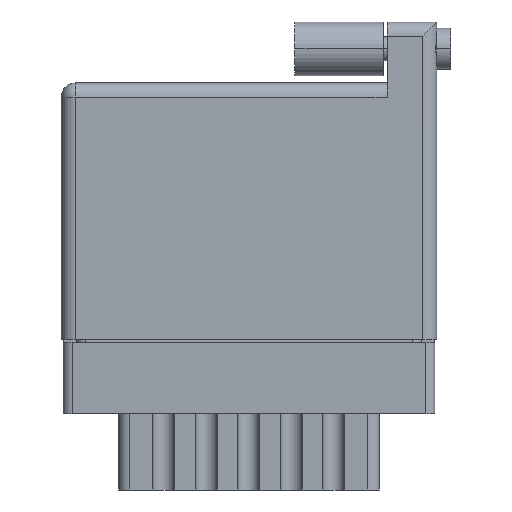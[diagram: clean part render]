
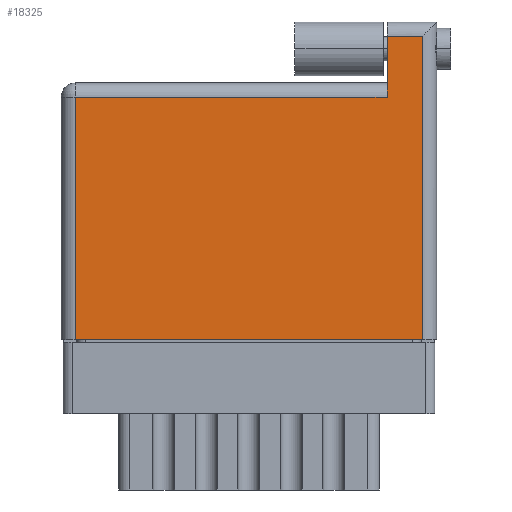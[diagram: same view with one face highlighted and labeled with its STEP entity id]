
A CAD part, front view. The second image highlights one B-rep face of the part: STEP entity #18325.
In plain terms, the highlighted face is planar.
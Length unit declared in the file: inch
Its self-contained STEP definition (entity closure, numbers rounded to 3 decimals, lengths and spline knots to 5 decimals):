
#205 = VECTOR ( 'NONE', #2744, 39.37008 ) ;
#471 = VERTEX_POINT ( 'NONE', #10055 ) ;
#605 = ORIENTED_EDGE ( 'NONE', *, *, #24249, .T. ) ;
#1663 = ORIENTED_EDGE ( 'NONE', *, *, #26194, .T. ) ;
#2381 = VECTOR ( 'NONE', #19100, 39.37008 ) ;
#2569 = LINE ( 'NONE', #28174, #23209 ) ;
#2744 = DIRECTION ( 'NONE',  ( -1., 0., 0. ) ) ;
#4416 = AXIS2_PLACEMENT_3D ( 'NONE', #20257, #10845, #27361 ) ;
#5084 = LINE ( 'NONE', #30230, #30281 ) ;
#5211 = LINE ( 'NONE', #28210, #205 ) ;
#5390 = CARTESIAN_POINT ( 'NONE',  ( 0.05, 0., 0. ) ) ;
#5573 = VERTEX_POINT ( 'NONE', #8824 ) ;
#6116 = EDGE_CURVE ( 'NONE', #5573, #471, #5084, .T. ) ;
#6940 = VECTOR ( 'NONE', #14784, 39.37008 ) ;
#7495 = DIRECTION ( 'NONE',  ( 0., 1., 0. ) ) ;
#7535 = EDGE_CURVE ( 'NONE', #26347, #5573, #5211, .T. ) ;
#7781 = CARTESIAN_POINT ( 'NONE',  ( 1.275, 0., 0. ) ) ;
#8824 = CARTESIAN_POINT ( 'NONE',  ( 1.15, 1.07, 0. ) ) ;
#9229 = DIRECTION ( 'NONE',  ( 0., -1., 0. ) ) ;
#9705 = CARTESIAN_POINT ( 'NONE',  ( 0., 0., 0. ) ) ;
#10055 = CARTESIAN_POINT ( 'NONE',  ( 1.15, 0.856, 0. ) ) ;
#10772 = VERTEX_POINT ( 'NONE', #20698 ) ;
#10845 = DIRECTION ( 'NONE',  ( 0., 0., -1. ) ) ;
#11033 = DIRECTION ( 'NONE',  ( -1., 0., 0. ) ) ;
#14148 = VECTOR ( 'NONE', #11033, 39.37008 ) ;
#14436 = ORIENTED_EDGE ( 'NONE', *, *, #6116, .T. ) ;
#14784 = DIRECTION ( 'NONE',  ( 0., -1., 0. ) ) ;
#14911 = VERTEX_POINT ( 'NONE', #7781 ) ;
#15650 = CARTESIAN_POINT ( 'NONE',  ( 0., 0.856, 0. ) ) ;
#16507 = VERTEX_POINT ( 'NONE', #23186 ) ;
#16800 = LINE ( 'NONE', #9705, #2381 ) ;
#16881 = CARTESIAN_POINT ( 'NONE',  ( 1.275, 1.07, 0. ) ) ;
#18325 = ADVANCED_FACE ( 'NONE', ( #19799 ), #24744, .F. ) ;
#18421 = LINE ( 'NONE', #15650, #14148 ) ;
#19100 = DIRECTION ( 'NONE',  ( 1., 0., 0. ) ) ;
#19799 = FACE_OUTER_BOUND ( 'NONE', #30518, .T. ) ;
#19894 = EDGE_CURVE ( 'NONE', #14911, #26347, #2569, .T. ) ;
#20257 = CARTESIAN_POINT ( 'NONE',  ( 0., 0.906, 0. ) ) ;
#20698 = CARTESIAN_POINT ( 'NONE',  ( 0.05, 0.856, 0. ) ) ;
#22997 = ORIENTED_EDGE ( 'NONE', *, *, #19894, .T. ) ;
#23186 = CARTESIAN_POINT ( 'NONE',  ( 0.05, 0., 0. ) ) ;
#23209 = VECTOR ( 'NONE', #7495, 39.37008 ) ;
#24249 = EDGE_CURVE ( 'NONE', #10772, #16507, #26507, .T. ) ;
#24744 = PLANE ( 'NONE',  #4416 ) ;
#26194 = EDGE_CURVE ( 'NONE', #471, #10772, #18421, .T. ) ;
#26277 = ORIENTED_EDGE ( 'NONE', *, *, #27428, .T. ) ;
#26347 = VERTEX_POINT ( 'NONE', #16881 ) ;
#26507 = LINE ( 'NONE', #5390, #6940 ) ;
#27361 = DIRECTION ( 'NONE',  ( -1., 0., 0. ) ) ;
#27428 = EDGE_CURVE ( 'NONE', #16507, #14911, #16800, .T. ) ;
#28174 = CARTESIAN_POINT ( 'NONE',  ( 1.275, 1.12, 0. ) ) ;
#28210 = CARTESIAN_POINT ( 'NONE',  ( 0., 1.07, 0. ) ) ;
#28671 = ORIENTED_EDGE ( 'NONE', *, *, #7535, .T. ) ;
#30230 = CARTESIAN_POINT ( 'NONE',  ( 1.15, 1.12, 0. ) ) ;
#30281 = VECTOR ( 'NONE', #9229, 39.37008 ) ;
#30518 = EDGE_LOOP ( 'NONE', ( #26277, #22997, #28671, #14436, #1663, #605 ) ) ;
